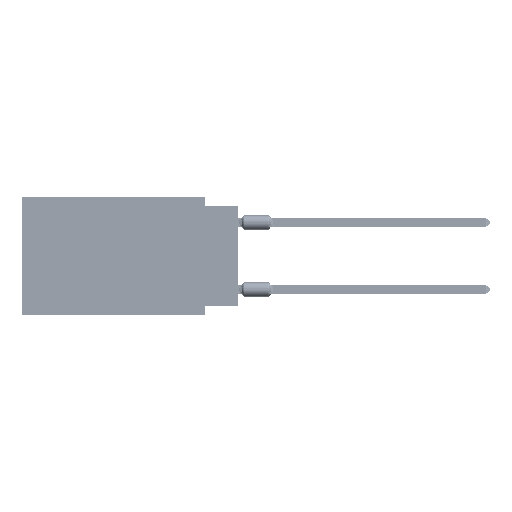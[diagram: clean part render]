
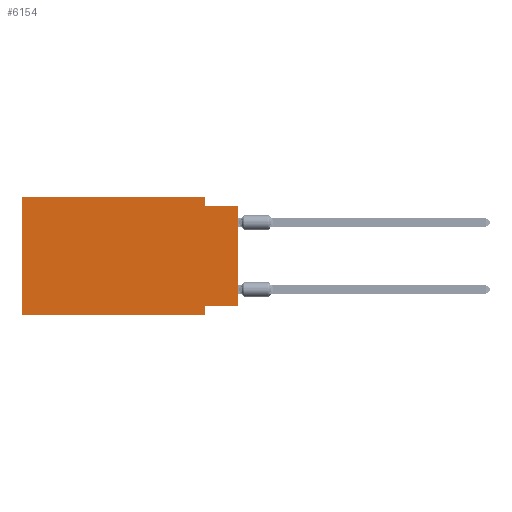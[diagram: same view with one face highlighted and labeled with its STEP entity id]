
A CAD part, left-side view. The second image highlights one B-rep face of the part: STEP entity #6154.
In plain terms, the highlighted planar face has unit normal (-1, 0, 0).
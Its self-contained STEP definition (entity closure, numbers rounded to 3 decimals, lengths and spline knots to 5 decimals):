
#559 = CARTESIAN_POINT ( 'NONE',  ( 0., 0.1, -0.35 ) ) ;
#1564 = LINE ( 'NONE', #101540, #15895 ) ;
#1679 = VERTEX_POINT ( 'NONE', #55915 ) ;
#6154 = ADVANCED_FACE ( 'NONE', ( #99207 ), #33053, .F. ) ;
#8220 = DIRECTION ( 'NONE',  ( 0., 1., 0. ) ) ;
#10518 = CARTESIAN_POINT ( 'NONE',  ( 0., 0.1, -0.025 ) ) ;
#11976 = CARTESIAN_POINT ( 'NONE',  ( 0., 0.645, 0. ) ) ;
#13314 = CARTESIAN_POINT ( 'NONE',  ( 0., 0.645, 0. ) ) ;
#13382 = VECTOR ( 'NONE', #33913, 39.37008 ) ;
#15895 = VECTOR ( 'NONE', #18232, 39.37008 ) ;
#15928 = EDGE_LOOP ( 'NONE', ( #73989, #78175, #17858, #27669, #48209, #40796, #101503, #19874 ) ) ;
#16937 = DIRECTION ( 'NONE',  ( 0., 0., -1. ) ) ;
#17858 = ORIENTED_EDGE ( 'NONE', *, *, #33186, .F. ) ;
#18232 = DIRECTION ( 'NONE',  ( 0., 0., -1. ) ) ;
#18884 = VERTEX_POINT ( 'NONE', #40157 ) ;
#19315 = VERTEX_POINT ( 'NONE', #76412 ) ;
#19388 = VECTOR ( 'NONE', #49770, 39.37008 ) ;
#19874 = ORIENTED_EDGE ( 'NONE', *, *, #85749, .F. ) ;
#19934 = CARTESIAN_POINT ( 'NONE',  ( 0., 0., 0. ) ) ;
#21411 = EDGE_CURVE ( 'NONE', #49735, #90796, #96107, .T. ) ;
#22533 = EDGE_CURVE ( 'NONE', #1679, #99090, #75393, .T. ) ;
#27669 = ORIENTED_EDGE ( 'NONE', *, *, #21411, .F. ) ;
#31556 = DIRECTION ( 'NONE',  ( 0., -1., 0. ) ) ;
#33053 = PLANE ( 'NONE',  #102120 ) ;
#33186 = EDGE_CURVE ( 'NONE', #90796, #75528, #1564, .T. ) ;
#33913 = DIRECTION ( 'NONE',  ( 0., 0., -1. ) ) ;
#40157 = CARTESIAN_POINT ( 'NONE',  ( 0., 0.1, -0.325 ) ) ;
#40796 = ORIENTED_EDGE ( 'NONE', *, *, #94619, .T. ) ;
#40922 = LINE ( 'NONE', #97383, #64858 ) ;
#41319 = VECTOR ( 'NONE', #102212, 39.37008 ) ;
#42910 = DIRECTION ( 'NONE',  ( 0., 0., 1. ) ) ;
#48209 = ORIENTED_EDGE ( 'NONE', *, *, #72657, .F. ) ;
#49735 = VERTEX_POINT ( 'NONE', #11976 ) ;
#49770 = DIRECTION ( 'NONE',  ( 0., -1., 0. ) ) ;
#50809 = CARTESIAN_POINT ( 'NONE',  ( 0., 0., -0.025 ) ) ;
#55915 = CARTESIAN_POINT ( 'NONE',  ( 0., 0., -0.325 ) ) ;
#57716 = CARTESIAN_POINT ( 'NONE',  ( 0., 0.1, 0. ) ) ;
#57796 = DIRECTION ( 'NONE',  ( 1., 0., 0. ) ) ;
#58816 = CARTESIAN_POINT ( 'NONE',  ( 0., 0.645, -0.35 ) ) ;
#59422 = CARTESIAN_POINT ( 'NONE',  ( 0., 0., -0.025 ) ) ;
#60611 = CARTESIAN_POINT ( 'NONE',  ( 0., 0.645, 0. ) ) ;
#64858 = VECTOR ( 'NONE', #98444, 39.37008 ) ;
#65850 = CARTESIAN_POINT ( 'NONE',  ( 0., 0.645, 0. ) ) ;
#67475 = LINE ( 'NONE', #50809, #19388 ) ;
#67648 = LINE ( 'NONE', #60611, #99283 ) ;
#72657 = EDGE_CURVE ( 'NONE', #80195, #49735, #67648, .T. ) ;
#73989 = ORIENTED_EDGE ( 'NONE', *, *, #22533, .T. ) ;
#75393 = LINE ( 'NONE', #19934, #41319 ) ;
#75528 = VERTEX_POINT ( 'NONE', #10518 ) ;
#75976 = EDGE_CURVE ( 'NONE', #18884, #19315, #82819, .T. ) ;
#76412 = CARTESIAN_POINT ( 'NONE',  ( 0., 0.1, -0.35 ) ) ;
#77240 = VECTOR ( 'NONE', #31556, 39.37008 ) ;
#78175 = ORIENTED_EDGE ( 'NONE', *, *, #85426, .F. ) ;
#80195 = VERTEX_POINT ( 'NONE', #58816 ) ;
#82819 = LINE ( 'NONE', #559, #13382 ) ;
#85426 = EDGE_CURVE ( 'NONE', #75528, #99090, #67475, .T. ) ;
#85749 = EDGE_CURVE ( 'NONE', #1679, #18884, #98568, .T. ) ;
#90796 = VERTEX_POINT ( 'NONE', #57716 ) ;
#94619 = EDGE_CURVE ( 'NONE', #80195, #19315, #40922, .T. ) ;
#94933 = VECTOR ( 'NONE', #8220, 39.37008 ) ;
#96107 = LINE ( 'NONE', #13314, #77240 ) ;
#97383 = CARTESIAN_POINT ( 'NONE',  ( 0., 0.645, -0.35 ) ) ;
#98444 = DIRECTION ( 'NONE',  ( 0., -1., 0. ) ) ;
#98568 = LINE ( 'NONE', #106104, #94933 ) ;
#99090 = VERTEX_POINT ( 'NONE', #59422 ) ;
#99207 = FACE_OUTER_BOUND ( 'NONE', #15928, .T. ) ;
#99283 = VECTOR ( 'NONE', #42910, 39.37008 ) ;
#101503 = ORIENTED_EDGE ( 'NONE', *, *, #75976, .F. ) ;
#101540 = CARTESIAN_POINT ( 'NONE',  ( 0., 0.1, 0. ) ) ;
#102120 = AXIS2_PLACEMENT_3D ( 'NONE', #65850, #57796, #16937 ) ;
#102212 = DIRECTION ( 'NONE',  ( 0., 0., 1. ) ) ;
#106104 = CARTESIAN_POINT ( 'NONE',  ( 0., 0., -0.325 ) ) ;
